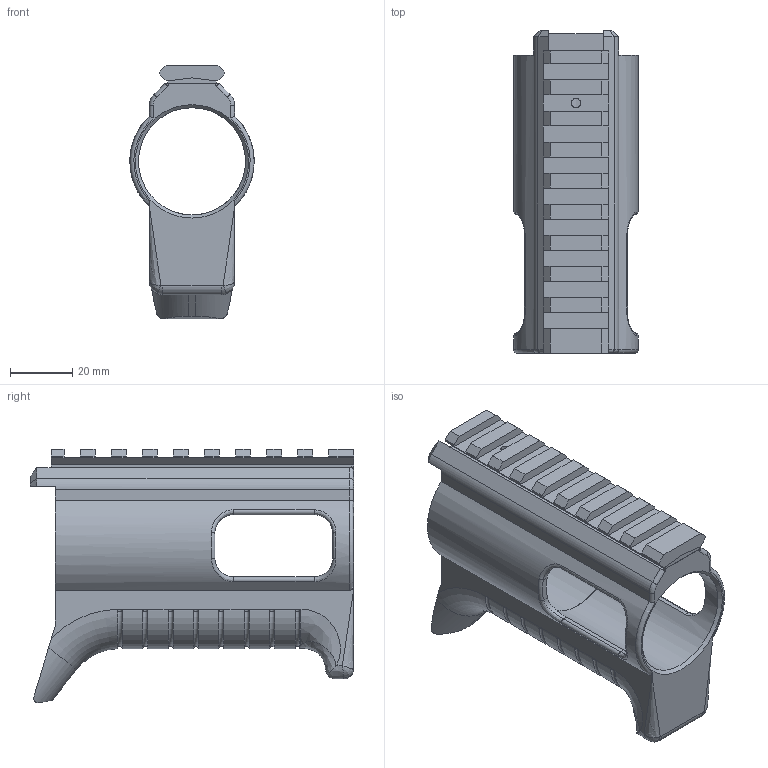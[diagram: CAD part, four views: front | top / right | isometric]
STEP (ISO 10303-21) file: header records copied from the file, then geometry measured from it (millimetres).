
FILE_DESCRIPTION(/* description */ (''),/* implementation_level */ '2;1');
FILE_NAME(/* name */ 'SG22 Handguard Release.step',/* time_stamp */ '2021-03-18T08:53:25-06:00',/* author */ (''),/* organization */ (''),/* preprocessor_version */ 'ST-DEVELOPER v18.1',/* originating_system */ 'Autodesk Translation Framework v9.10.0.1330',/* authorisation */ '');
FILE_SCHEMA (('AUTOMOTIVE_DESIGN { 1 0 10303 214 3 1 1 }'));
Length unit declared in the file: millimetre
Products named in the file (1): Brace V2
Bounding box: 40 x 104 x 81.71 mm (x, y, z)
Volume: 85152.4 mm3; surface area: 30352.3 mm2
Topology: 1 solids, 1 shells, 277 faces, 690 edges, 405 vertices
Faces by surface type: plane 153, cylinder 56, bspline 38, torus 26, cone 4
Full cylindrical faces by diameter (mm): 34.5 x1, 36.5 x1
Entity records: 11483 total; most frequent: CARTESIAN_POINT 5223, ORIENTED_EDGE 1368, DIRECTION 1161, EDGE_CURVE 684, LINE 411, VECTOR 411, VERTEX_POINT 405, AXIS2_PLACEMENT_3D 375
